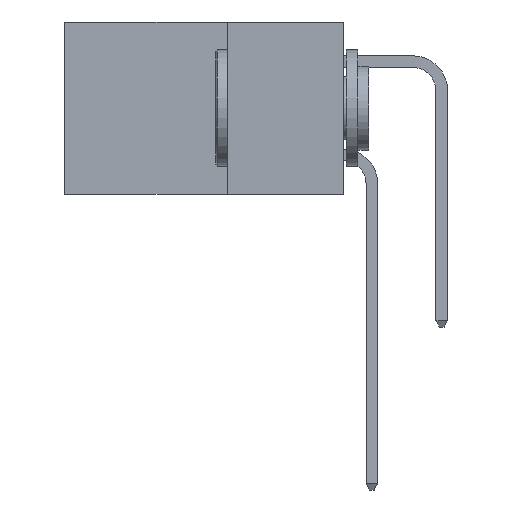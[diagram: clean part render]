
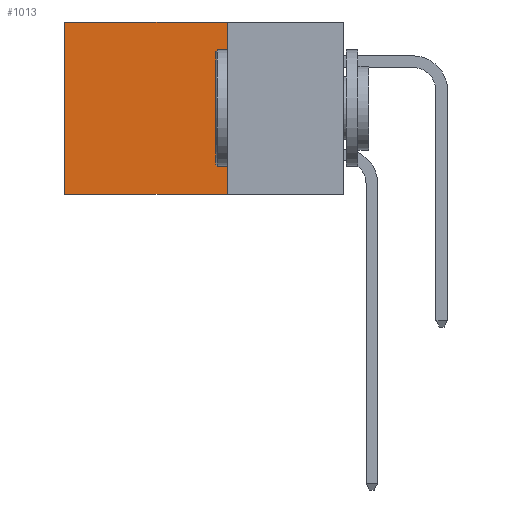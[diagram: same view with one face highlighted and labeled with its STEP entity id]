
A CAD part, left-side view. The second image highlights one B-rep face of the part: STEP entity #1013.
In plain terms, the highlighted planar face has unit normal (-1, 0, 0).
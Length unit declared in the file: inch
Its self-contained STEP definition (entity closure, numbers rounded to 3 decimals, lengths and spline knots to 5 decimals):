
#118 = VECTOR ( 'NONE', #11881, 39.37008 ) ;
#1013 = ADVANCED_FACE ( 'NONE', ( #10970 ), #12635, .F. ) ;
#1139 = EDGE_CURVE ( 'NONE', #10254, #4240, #10235, .T. ) ;
#1496 = EDGE_CURVE ( 'NONE', #5385, #4240, #10955, .T. ) ;
#1626 = VECTOR ( 'NONE', #14159, 39.37008 ) ;
#2330 = CARTESIAN_POINT ( 'NONE',  ( 0.2615, 0.25, -0.37 ) ) ;
#3457 = VERTEX_POINT ( 'NONE', #13823 ) ;
#3636 = EDGE_CURVE ( 'NONE', #3457, #5385, #13107, .T. ) ;
#4240 = VERTEX_POINT ( 'NONE', #13987 ) ;
#4250 = AXIS2_PLACEMENT_3D ( 'NONE', #2330, #8497, #6432 ) ;
#4746 = EDGE_CURVE ( 'NONE', #3457, #10254, #6498, .T. ) ;
#5033 = ORIENTED_EDGE ( 'NONE', *, *, #1496, .F. ) ;
#5288 = CARTESIAN_POINT ( 'NONE',  ( 0.2615, 0.25, -0.37 ) ) ;
#5385 = VERTEX_POINT ( 'NONE', #5288 ) ;
#6101 = CARTESIAN_POINT ( 'NONE',  ( 0.2615, 0.6, 0. ) ) ;
#6130 = CARTESIAN_POINT ( 'NONE',  ( 0.2615, 0.6, -0.37 ) ) ;
#6432 = DIRECTION ( 'NONE',  ( 0., 0., -1. ) ) ;
#6498 = LINE ( 'NONE', #10403, #12512 ) ;
#8094 = CARTESIAN_POINT ( 'NONE',  ( 0.2615, 0.25, -0.37 ) ) ;
#8497 = DIRECTION ( 'NONE',  ( 1., 0., 0. ) ) ;
#9384 = ORIENTED_EDGE ( 'NONE', *, *, #4746, .T. ) ;
#9949 = VECTOR ( 'NONE', #10347, 39.37008 ) ;
#10235 = LINE ( 'NONE', #6130, #118 ) ;
#10254 = VERTEX_POINT ( 'NONE', #6101 ) ;
#10347 = DIRECTION ( 'NONE',  ( 0., 0., -1. ) ) ;
#10398 = DIRECTION ( 'NONE',  ( 0., 1., 0. ) ) ;
#10403 = CARTESIAN_POINT ( 'NONE',  ( 0.2615, 0.25, 0. ) ) ;
#10955 = LINE ( 'NONE', #8094, #1626 ) ;
#10970 = FACE_OUTER_BOUND ( 'NONE', #14812, .T. ) ;
#11179 = CARTESIAN_POINT ( 'NONE',  ( 0.2615, 0.25, -0.37 ) ) ;
#11400 = ORIENTED_EDGE ( 'NONE', *, *, #3636, .F. ) ;
#11881 = DIRECTION ( 'NONE',  ( 0., 0., -1. ) ) ;
#12175 = ORIENTED_EDGE ( 'NONE', *, *, #1139, .T. ) ;
#12512 = VECTOR ( 'NONE', #10398, 39.37008 ) ;
#12635 = PLANE ( 'NONE',  #4250 ) ;
#13107 = LINE ( 'NONE', #11179, #9949 ) ;
#13823 = CARTESIAN_POINT ( 'NONE',  ( 0.2615, 0.25, 0. ) ) ;
#13987 = CARTESIAN_POINT ( 'NONE',  ( 0.2615, 0.6, -0.37 ) ) ;
#14159 = DIRECTION ( 'NONE',  ( 0., 1., 0. ) ) ;
#14812 = EDGE_LOOP ( 'NONE', ( #12175, #5033, #11400, #9384 ) ) ;
